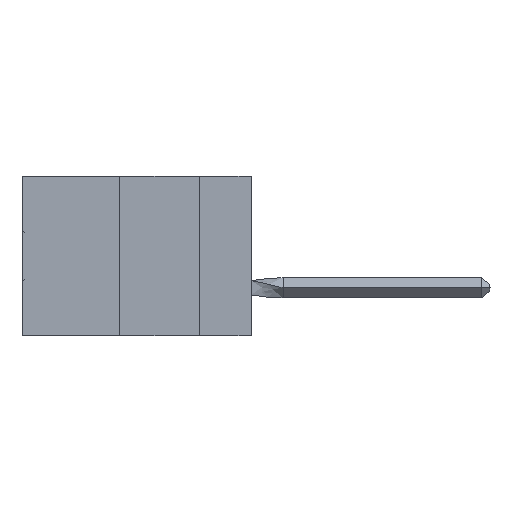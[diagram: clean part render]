
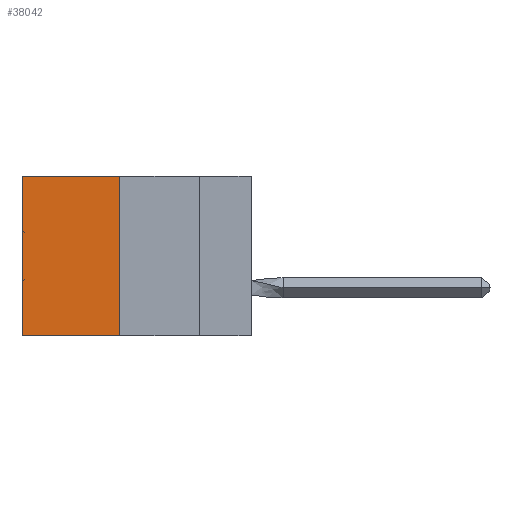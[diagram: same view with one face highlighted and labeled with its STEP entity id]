
A CAD part, left-side view. The second image highlights one B-rep face of the part: STEP entity #38042.
In plain terms, the highlighted planar face has unit normal (-1, 0, 0).
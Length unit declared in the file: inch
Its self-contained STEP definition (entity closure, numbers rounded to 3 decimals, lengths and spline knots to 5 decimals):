
#519 = VERTEX_POINT ( 'NONE', #42244 ) ;
#705 = CARTESIAN_POINT ( 'NONE',  ( 0.305, 0.72, 0. ) ) ;
#952 = ORIENTED_EDGE ( 'NONE', *, *, #50951, .T. ) ;
#1325 = DIRECTION ( 'NONE',  ( 0., 1., 0. ) ) ;
#2760 = CARTESIAN_POINT ( 'NONE',  ( 0.305, 0.413, 0. ) ) ;
#3256 = DIRECTION ( 'NONE',  ( 0., 0., -1. ) ) ;
#7905 = VECTOR ( 'NONE', #27705, 39.37008 ) ;
#10804 = AXIS2_PLACEMENT_3D ( 'NONE', #50016, #41718, #12600 ) ;
#12268 = VECTOR ( 'NONE', #30879, 39.37008 ) ;
#12600 = DIRECTION ( 'NONE',  ( 0., 0., -1. ) ) ;
#13054 = VECTOR ( 'NONE', #1325, 39.37008 ) ;
#16737 = EDGE_CURVE ( 'NONE', #34390, #49095, #26991, .T. ) ;
#18933 = CARTESIAN_POINT ( 'NONE',  ( 0.305, 0.413, -0.5 ) ) ;
#25408 = LINE ( 'NONE', #52505, #12268 ) ;
#26123 = VERTEX_POINT ( 'NONE', #705 ) ;
#26991 = LINE ( 'NONE', #18933, #42662 ) ;
#27596 = LINE ( 'NONE', #2760, #7905 ) ;
#27705 = DIRECTION ( 'NONE',  ( 0., 1., 0. ) ) ;
#29375 = EDGE_CURVE ( 'NONE', #26123, #519, #25408, .T. ) ;
#30879 = DIRECTION ( 'NONE',  ( 0., 0., -1. ) ) ;
#33116 = CARTESIAN_POINT ( 'NONE',  ( 0.305, 0.413, -0.5 ) ) ;
#34390 = VERTEX_POINT ( 'NONE', #36474 ) ;
#35364 = LINE ( 'NONE', #47137, #13054 ) ;
#35705 = EDGE_CURVE ( 'NONE', #49095, #519, #35364, .T. ) ;
#36474 = CARTESIAN_POINT ( 'NONE',  ( 0.305, 0.413, 0. ) ) ;
#38042 = ADVANCED_FACE ( 'NONE', ( #53455 ), #41538, .F. ) ;
#38243 = EDGE_LOOP ( 'NONE', ( #44529, #49822, #42443, #952 ) ) ;
#41538 = PLANE ( 'NONE',  #10804 ) ;
#41718 = DIRECTION ( 'NONE',  ( 1., 0., 0. ) ) ;
#42244 = CARTESIAN_POINT ( 'NONE',  ( 0.305, 0.72, -0.5 ) ) ;
#42443 = ORIENTED_EDGE ( 'NONE', *, *, #16737, .F. ) ;
#42662 = VECTOR ( 'NONE', #3256, 39.37008 ) ;
#44529 = ORIENTED_EDGE ( 'NONE', *, *, #29375, .T. ) ;
#47137 = CARTESIAN_POINT ( 'NONE',  ( 0.305, 0.413, -0.5 ) ) ;
#49095 = VERTEX_POINT ( 'NONE', #33116 ) ;
#49822 = ORIENTED_EDGE ( 'NONE', *, *, #35705, .F. ) ;
#50016 = CARTESIAN_POINT ( 'NONE',  ( 0.305, 0.413, -0.5 ) ) ;
#50951 = EDGE_CURVE ( 'NONE', #34390, #26123, #27596, .T. ) ;
#52505 = CARTESIAN_POINT ( 'NONE',  ( 0.305, 0.72, -0.5 ) ) ;
#53455 = FACE_OUTER_BOUND ( 'NONE', #38243, .T. ) ;
